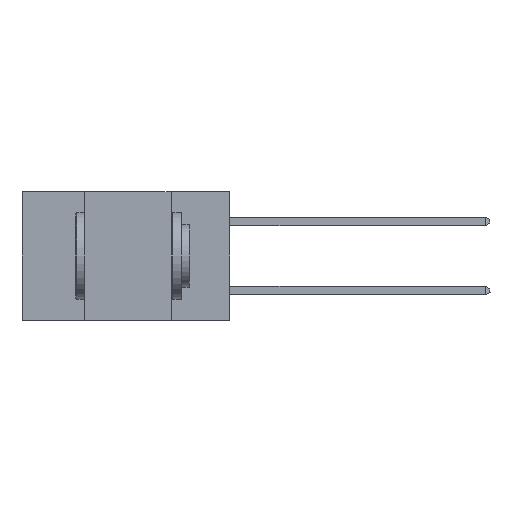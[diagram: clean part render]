
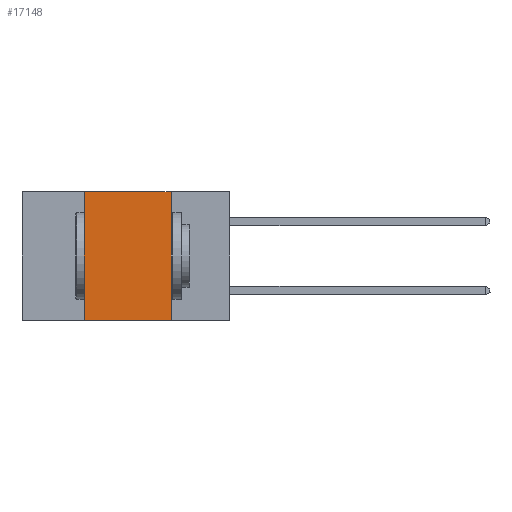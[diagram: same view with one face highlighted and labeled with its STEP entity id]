
A CAD part, left-side view. The second image highlights one B-rep face of the part: STEP entity #17148.
In plain terms, the highlighted planar face has unit normal (-1, 0, 0).
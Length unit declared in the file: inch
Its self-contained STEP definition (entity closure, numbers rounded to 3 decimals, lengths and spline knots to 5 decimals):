
#676 = VERTEX_POINT ( 'NONE', #19983 ) ;
#780 = EDGE_CURVE ( 'NONE', #18459, #676, #21256, .T. ) ;
#877 = CARTESIAN_POINT ( 'NONE',  ( 0., 0.17, 0. ) ) ;
#1689 = DIRECTION ( 'NONE',  ( 0., -1., 0. ) ) ;
#1995 = AXIS2_PLACEMENT_3D ( 'NONE', #8934, #7386, #4187 ) ;
#2019 = VECTOR ( 'NONE', #16804, 39.37008 ) ;
#2887 = CARTESIAN_POINT ( 'NONE',  ( 0., 0.42, 0. ) ) ;
#3330 = CARTESIAN_POINT ( 'NONE',  ( 0., 0.6, -0.37 ) ) ;
#4187 = DIRECTION ( 'NONE',  ( 0., 0., -1. ) ) ;
#5272 = VERTEX_POINT ( 'NONE', #11289 ) ;
#6537 = FACE_OUTER_BOUND ( 'NONE', #15690, .T. ) ;
#7188 = CARTESIAN_POINT ( 'NONE',  ( 0., 0.42, 0. ) ) ;
#7314 = EDGE_CURVE ( 'NONE', #18440, #5272, #19963, .T. ) ;
#7386 = DIRECTION ( 'NONE',  ( 1., 0., 0. ) ) ;
#8934 = CARTESIAN_POINT ( 'NONE',  ( 0., 0.6, 0. ) ) ;
#10680 = DIRECTION ( 'NONE',  ( 0., 0., -1. ) ) ;
#11289 = CARTESIAN_POINT ( 'NONE',  ( 0., 0.17, -0.37 ) ) ;
#12293 = PLANE ( 'NONE',  #1995 ) ;
#12817 = DIRECTION ( 'NONE',  ( 0., 0., 1. ) ) ;
#13308 = ORIENTED_EDGE ( 'NONE', *, *, #21348, .F. ) ;
#14132 = ORIENTED_EDGE ( 'NONE', *, *, #7314, .T. ) ;
#14270 = EDGE_CURVE ( 'NONE', #676, #5272, #18891, .T. ) ;
#14493 = VECTOR ( 'NONE', #1689, 39.37008 ) ;
#15064 = ORIENTED_EDGE ( 'NONE', *, *, #14270, .F. ) ;
#15196 = VECTOR ( 'NONE', #12817, 39.37008 ) ;
#15426 = CARTESIAN_POINT ( 'NONE',  ( 0., 0.42, -0.37 ) ) ;
#15690 = EDGE_LOOP ( 'NONE', ( #15064, #20462, #13308, #14132 ) ) ;
#16804 = DIRECTION ( 'NONE',  ( 0., -1., 0. ) ) ;
#17148 = ADVANCED_FACE ( 'NONE', ( #6537 ), #12293, .F. ) ;
#17569 = VECTOR ( 'NONE', #10680, 39.37008 ) ;
#18392 = CARTESIAN_POINT ( 'NONE',  ( 0., 0.6, 0. ) ) ;
#18440 = VERTEX_POINT ( 'NONE', #15426 ) ;
#18459 = VERTEX_POINT ( 'NONE', #7188 ) ;
#18891 = LINE ( 'NONE', #877, #17569 ) ;
#19963 = LINE ( 'NONE', #3330, #14493 ) ;
#19983 = CARTESIAN_POINT ( 'NONE',  ( 0., 0.17, 0. ) ) ;
#20388 = LINE ( 'NONE', #2887, #15196 ) ;
#20462 = ORIENTED_EDGE ( 'NONE', *, *, #780, .F. ) ;
#21256 = LINE ( 'NONE', #18392, #2019 ) ;
#21348 = EDGE_CURVE ( 'NONE', #18440, #18459, #20388, .T. ) ;
